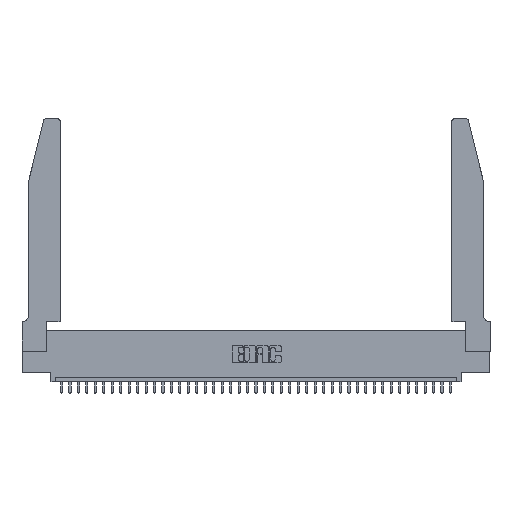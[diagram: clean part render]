
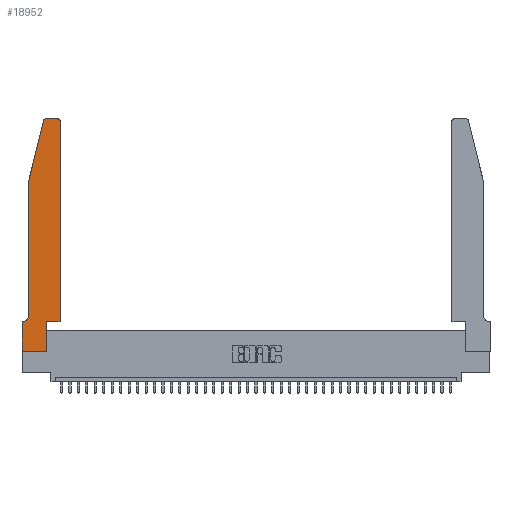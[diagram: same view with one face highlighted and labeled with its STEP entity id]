
A CAD part, top view. The second image highlights one B-rep face of the part: STEP entity #18952.
In plain terms, the highlighted planar face has unit normal (0, 0, 1).
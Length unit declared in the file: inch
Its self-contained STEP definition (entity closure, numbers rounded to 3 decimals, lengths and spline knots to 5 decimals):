
#457 = ORIENTED_EDGE ( 'NONE', *, *, #12939, .T. ) ;
#549 = DIRECTION ( 'NONE',  ( 1., 0., 0. ) ) ;
#694 = EDGE_CURVE ( 'NONE', #10573, #31259, #36470, .T. ) ;
#743 = AXIS2_PLACEMENT_3D ( 'NONE', #31657, #18890, #549 ) ;
#1830 = VECTOR ( 'NONE', #37364, 39.37008 ) ;
#2136 = ORIENTED_EDGE ( 'NONE', *, *, #21793, .T. ) ;
#2163 = ORIENTED_EDGE ( 'NONE', *, *, #39127, .T. ) ;
#3352 = CARTESIAN_POINT ( 'NONE',  ( 0.0055, 0.35, 0.37 ) ) ;
#3652 = LINE ( 'NONE', #5556, #24726 ) ;
#3691 = DIRECTION ( 'NONE',  ( 1., 0., 0. ) ) ;
#4851 = LINE ( 'NONE', #18001, #7705 ) ;
#5222 = VECTOR ( 'NONE', #8415, 39.37008 ) ;
#5458 = CARTESIAN_POINT ( 'NONE',  ( 0.0755, 2., 0.37 ) ) ;
#5552 = ORIENTED_EDGE ( 'NONE', *, *, #23133, .T. ) ;
#5556 = CARTESIAN_POINT ( 'NONE',  ( 0.4505, 0.35, 0.37 ) ) ;
#5992 = VECTOR ( 'NONE', #18981, 39.37008 ) ;
#6231 = VERTEX_POINT ( 'NONE', #10831 ) ;
#6915 = CARTESIAN_POINT ( 'NONE',  ( 0.4505, 0.35, 0.37 ) ) ;
#7258 = CARTESIAN_POINT ( 'NONE',  ( 0., 0., 0.37 ) ) ;
#7378 = VERTEX_POINT ( 'NONE', #29831 ) ;
#7462 = AXIS2_PLACEMENT_3D ( 'NONE', #36168, #26524, #35904 ) ;
#7705 = VECTOR ( 'NONE', #33534, 39.37008 ) ;
#7831 = ORIENTED_EDGE ( 'NONE', *, *, #30941, .T. ) ;
#8415 = DIRECTION ( 'NONE',  ( 0., -1., 0. ) ) ;
#8784 = LINE ( 'NONE', #13993, #38943 ) ;
#8859 = ORIENTED_EDGE ( 'NONE', *, *, #20331, .T. ) ;
#9140 = VECTOR ( 'NONE', #38523, 39.37008 ) ;
#9332 = CARTESIAN_POINT ( 'NONE',  ( 0.284, 2.75, 0.37 ) ) ;
#10030 = CARTESIAN_POINT ( 'NONE',  ( 0.0055, 0.42, 0.37 ) ) ;
#10085 = DIRECTION ( 'NONE',  ( 0., 1., 0. ) ) ;
#10573 = VERTEX_POINT ( 'NONE', #21390 ) ;
#10587 = DIRECTION ( 'NONE',  ( -1., 0., 0. ) ) ;
#10831 = CARTESIAN_POINT ( 'NONE',  ( 0.4205, 2.75, 0.37 ) ) ;
#12939 = EDGE_CURVE ( 'NONE', #35802, #38171, #17374, .T. ) ;
#13265 = DIRECTION ( 'NONE',  ( 0., 0., -1. ) ) ;
#13618 = EDGE_LOOP ( 'NONE', ( #31215, #457, #17504, #2163, #17996, #30752, #7831, #35929, #15841, #5552, #2136, #8859 ) ) ;
#13993 = CARTESIAN_POINT ( 'NONE',  ( 0.0755, 2., 0.37 ) ) ;
#14074 = LINE ( 'NONE', #6915, #5992 ) ;
#14502 = CARTESIAN_POINT ( 'NONE',  ( 0.2865, 0., 0.37 ) ) ;
#15323 = AXIS2_PLACEMENT_3D ( 'NONE', #19358, #22017, #3691 ) ;
#15841 = ORIENTED_EDGE ( 'NONE', *, *, #33921, .T. ) ;
#16374 = VERTEX_POINT ( 'NONE', #5458 ) ;
#17119 = CARTESIAN_POINT ( 'NONE',  ( 0.0755, 2., 0.37 ) ) ;
#17370 = DIRECTION ( 'NONE',  ( -0.239, -0.971, 0. ) ) ;
#17374 = CIRCLE ( 'NONE', #7462, 0.03 ) ;
#17504 = ORIENTED_EDGE ( 'NONE', *, *, #37807, .T. ) ;
#17996 = ORIENTED_EDGE ( 'NONE', *, *, #30264, .T. ) ;
#18001 = CARTESIAN_POINT ( 'NONE',  ( 0.0755, 0.35, 0.37 ) ) ;
#18254 = FACE_OUTER_BOUND ( 'NONE', #13618, .T. ) ;
#18890 = DIRECTION ( 'NONE',  ( 0., 0., 1. ) ) ;
#18952 = ADVANCED_FACE ( 'NONE', ( #18254 ), #22140, .T. ) ;
#18981 = DIRECTION ( 'NONE',  ( 1., 0., 0. ) ) ;
#19358 = CARTESIAN_POINT ( 'NONE',  ( 0., 0.35, 0.37 ) ) ;
#19565 = CIRCLE ( 'NONE', #743, 0.03 ) ;
#20331 = EDGE_CURVE ( 'NONE', #21818, #6231, #19565, .T. ) ;
#20824 = CARTESIAN_POINT ( 'NONE',  ( 0.4505, 2.72, 0.37 ) ) ;
#21390 = CARTESIAN_POINT ( 'NONE',  ( 0., 0., 0.37 ) ) ;
#21793 = EDGE_CURVE ( 'NONE', #39294, #21818, #3652, .T. ) ;
#21818 = VERTEX_POINT ( 'NONE', #20824 ) ;
#21824 = CARTESIAN_POINT ( 'NONE',  ( 0., 0., 0.37 ) ) ;
#22017 = DIRECTION ( 'NONE',  ( 0., 0., 1. ) ) ;
#22140 = PLANE ( 'NONE',  #15323 ) ;
#23133 = EDGE_CURVE ( 'NONE', #39501, #39294, #14074, .T. ) ;
#23390 = VERTEX_POINT ( 'NONE', #3352 ) ;
#24217 = CARTESIAN_POINT ( 'NONE',  ( 0.4505, 0.35, 0.37 ) ) ;
#24232 = VECTOR ( 'NONE', #25530, 39.37008 ) ;
#24726 = VECTOR ( 'NONE', #26962, 39.37008 ) ;
#24779 = LINE ( 'NONE', #25316, #1830 ) ;
#24793 = LINE ( 'NONE', #17119, #5222 ) ;
#25268 = AXIS2_PLACEMENT_3D ( 'NONE', #10030, #13265, #10587 ) ;
#25316 = CARTESIAN_POINT ( 'NONE',  ( 0.2605, 2.75, 0.37 ) ) ;
#25502 = CARTESIAN_POINT ( 'NONE',  ( 0.2865, 0.35, 0.37 ) ) ;
#25530 = DIRECTION ( 'NONE',  ( 0., -1., 0. ) ) ;
#25726 = VERTEX_POINT ( 'NONE', #32221 ) ;
#25739 = CARTESIAN_POINT ( 'NONE',  ( 0.2865, 0.35, 0.37 ) ) ;
#26524 = DIRECTION ( 'NONE',  ( 0., 0., 1. ) ) ;
#26962 = DIRECTION ( 'NONE',  ( 0., 1., 0. ) ) ;
#27614 = CIRCLE ( 'NONE', #25268, 0.07 ) ;
#27705 = VECTOR ( 'NONE', #10085, 39.37008 ) ;
#29831 = CARTESIAN_POINT ( 'NONE',  ( 0.0755, 0.42, 0.37 ) ) ;
#30264 = EDGE_CURVE ( 'NONE', #7378, #23390, #27614, .T. ) ;
#30752 = ORIENTED_EDGE ( 'NONE', *, *, #32975, .T. ) ;
#30941 = EDGE_CURVE ( 'NONE', #25726, #10573, #37108, .T. ) ;
#31215 = ORIENTED_EDGE ( 'NONE', *, *, #34529, .T. ) ;
#31259 = VERTEX_POINT ( 'NONE', #14502 ) ;
#31657 = CARTESIAN_POINT ( 'NONE',  ( 0.4205, 2.72, 0.37 ) ) ;
#32221 = CARTESIAN_POINT ( 'NONE',  ( 0., 0.35, 0.37 ) ) ;
#32975 = EDGE_CURVE ( 'NONE', #23390, #25726, #4851, .T. ) ;
#33534 = DIRECTION ( 'NONE',  ( -1., 0., 0. ) ) ;
#33921 = EDGE_CURVE ( 'NONE', #31259, #39501, #38726, .T. ) ;
#34529 = EDGE_CURVE ( 'NONE', #6231, #35802, #24779, .T. ) ;
#35802 = VERTEX_POINT ( 'NONE', #9332 ) ;
#35904 = DIRECTION ( 'NONE',  ( 1., 0., 0. ) ) ;
#35929 = ORIENTED_EDGE ( 'NONE', *, *, #694, .T. ) ;
#36168 = CARTESIAN_POINT ( 'NONE',  ( 0.284, 2.72, 0.37 ) ) ;
#36470 = LINE ( 'NONE', #21824, #9140 ) ;
#36869 = CARTESIAN_POINT ( 'NONE',  ( 0.25487, 2.72718, 0.37 ) ) ;
#37108 = LINE ( 'NONE', #7258, #24232 ) ;
#37364 = DIRECTION ( 'NONE',  ( -1., 0., 0. ) ) ;
#37807 = EDGE_CURVE ( 'NONE', #38171, #16374, #8784, .T. ) ;
#38171 = VERTEX_POINT ( 'NONE', #36869 ) ;
#38523 = DIRECTION ( 'NONE',  ( 1., 0., 0. ) ) ;
#38726 = LINE ( 'NONE', #25502, #27705 ) ;
#38943 = VECTOR ( 'NONE', #17370, 39.37008 ) ;
#39127 = EDGE_CURVE ( 'NONE', #16374, #7378, #24793, .T. ) ;
#39294 = VERTEX_POINT ( 'NONE', #24217 ) ;
#39501 = VERTEX_POINT ( 'NONE', #25739 ) ;
